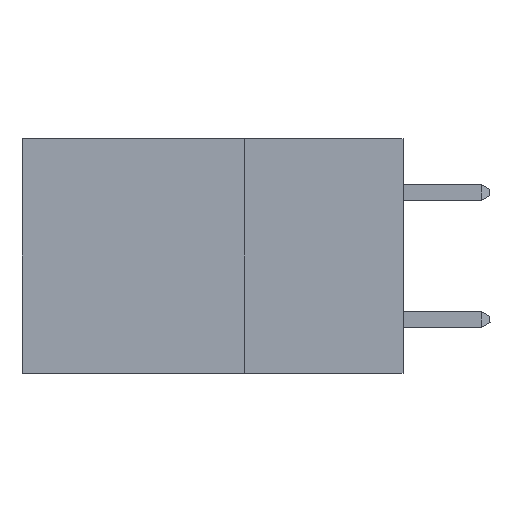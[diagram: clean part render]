
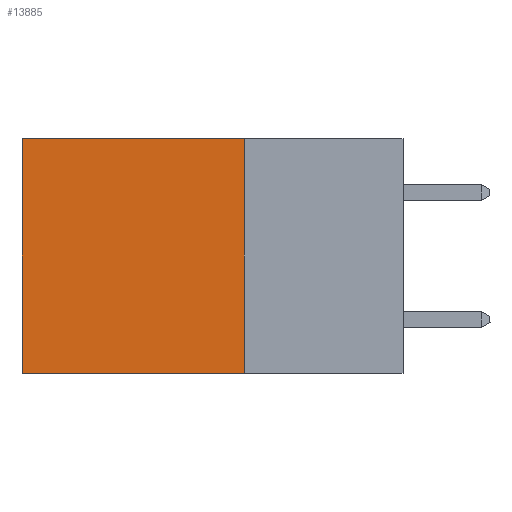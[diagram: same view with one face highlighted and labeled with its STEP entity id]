
A CAD part, left-side view. The second image highlights one B-rep face of the part: STEP entity #13885.
In plain terms, the highlighted planar face has unit normal (-1, 0, 0).
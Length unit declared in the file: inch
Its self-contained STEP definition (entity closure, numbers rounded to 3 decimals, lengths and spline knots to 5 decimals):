
#567 = DIRECTION ( 'NONE',  ( 0., 0., -1. ) ) ;
#1712 = CARTESIAN_POINT ( 'NONE',  ( 0.2875, 0.25, 0. ) ) ;
#3672 = LINE ( 'NONE', #6517, #24305 ) ;
#4427 = DIRECTION ( 'NONE',  ( 0., 0., -1. ) ) ;
#5527 = CARTESIAN_POINT ( 'NONE',  ( 0.2875, 0.6, 0. ) ) ;
#5741 = ORIENTED_EDGE ( 'NONE', *, *, #9670, .T. ) ;
#6264 = AXIS2_PLACEMENT_3D ( 'NONE', #1712, #19682, #13344 ) ;
#6517 = CARTESIAN_POINT ( 'NONE',  ( 0.2875, 0.25, 0. ) ) ;
#6656 = VECTOR ( 'NONE', #22006, 39.37008 ) ;
#7267 = CARTESIAN_POINT ( 'NONE',  ( 0.2875, 0.6, 0. ) ) ;
#8292 = CARTESIAN_POINT ( 'NONE',  ( 0.2875, 0.25, 0. ) ) ;
#8765 = ORIENTED_EDGE ( 'NONE', *, *, #22510, .F. ) ;
#9581 = EDGE_LOOP ( 'NONE', ( #5741, #24725, #8765, #16198 ) ) ;
#9670 = EDGE_CURVE ( 'NONE', #14325, #25731, #20583, .T. ) ;
#10518 = CARTESIAN_POINT ( 'NONE',  ( 0.2875, 0.25, -0.37 ) ) ;
#11562 = PLANE ( 'NONE',  #6264 ) ;
#12986 = EDGE_CURVE ( 'NONE', #25416, #14325, #23547, .T. ) ;
#13344 = DIRECTION ( 'NONE',  ( 0., 0., -1. ) ) ;
#13403 = EDGE_CURVE ( 'NONE', #19265, #25731, #23228, .T. ) ;
#13885 = ADVANCED_FACE ( 'NONE', ( #17525 ), #11562, .F. ) ;
#14325 = VERTEX_POINT ( 'NONE', #7267 ) ;
#15680 = DIRECTION ( 'NONE',  ( 0., 1., 0. ) ) ;
#15691 = CARTESIAN_POINT ( 'NONE',  ( 0.2875, 0.25, 0. ) ) ;
#16198 = ORIENTED_EDGE ( 'NONE', *, *, #12986, .T. ) ;
#17525 = FACE_OUTER_BOUND ( 'NONE', #9581, .T. ) ;
#18864 = VECTOR ( 'NONE', #15680, 39.37008 ) ;
#19265 = VERTEX_POINT ( 'NONE', #10518 ) ;
#19682 = DIRECTION ( 'NONE',  ( 1., 0., 0. ) ) ;
#20583 = LINE ( 'NONE', #5527, #24651 ) ;
#22006 = DIRECTION ( 'NONE',  ( 0., 1., 0. ) ) ;
#22193 = CARTESIAN_POINT ( 'NONE',  ( 0.2875, 0.25, -0.37 ) ) ;
#22510 = EDGE_CURVE ( 'NONE', #25416, #19265, #3672, .T. ) ;
#23228 = LINE ( 'NONE', #22193, #6656 ) ;
#23547 = LINE ( 'NONE', #8292, #18864 ) ;
#24305 = VECTOR ( 'NONE', #4427, 39.37008 ) ;
#24651 = VECTOR ( 'NONE', #567, 39.37008 ) ;
#24666 = CARTESIAN_POINT ( 'NONE',  ( 0.2875, 0.6, -0.37 ) ) ;
#24725 = ORIENTED_EDGE ( 'NONE', *, *, #13403, .F. ) ;
#25416 = VERTEX_POINT ( 'NONE', #15691 ) ;
#25731 = VERTEX_POINT ( 'NONE', #24666 ) ;
